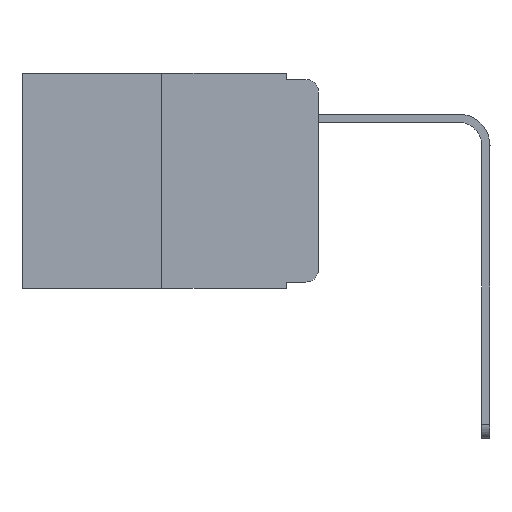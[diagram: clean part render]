
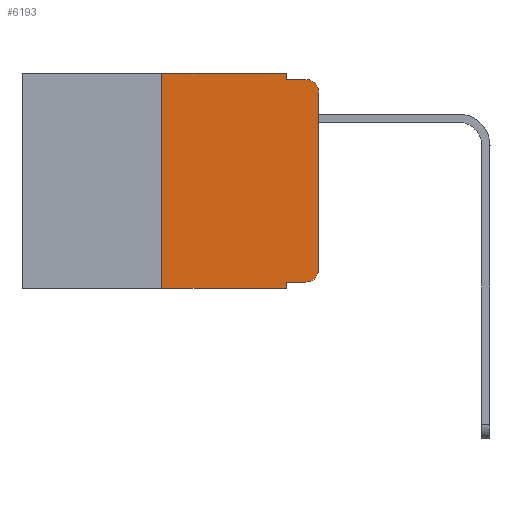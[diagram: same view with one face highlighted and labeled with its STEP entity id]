
A CAD part, left-side view. The second image highlights one B-rep face of the part: STEP entity #6193.
In plain terms, the highlighted planar face has unit normal (-1, 0, 0).
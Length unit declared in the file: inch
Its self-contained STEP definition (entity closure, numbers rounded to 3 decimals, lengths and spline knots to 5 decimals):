
#42 = LINE ( 'NONE', #4473, #7339 ) ;
#192 = CARTESIAN_POINT ( 'NONE',  ( 0., 0., -0.313 ) ) ;
#453 = DIRECTION ( 'NONE',  ( 0., -1., 0. ) ) ;
#806 = PLANE ( 'NONE',  #13889 ) ;
#850 = EDGE_CURVE ( 'NONE', #6566, #1438, #13291, .T. ) ;
#931 = DIRECTION ( 'NONE',  ( 0., 0., -1. ) ) ;
#1097 = ORIENTED_EDGE ( 'NONE', *, *, #3988, .F. ) ;
#1257 = ORIENTED_EDGE ( 'NONE', *, *, #9052, .F. ) ;
#1425 = ORIENTED_EDGE ( 'NONE', *, *, #13205, .F. ) ;
#1438 = VERTEX_POINT ( 'NONE', #192 ) ;
#2162 = CARTESIAN_POINT ( 'NONE',  ( 0., 0.051, -0.333 ) ) ;
#2212 = VERTEX_POINT ( 'NONE', #12755 ) ;
#2245 = CARTESIAN_POINT ( 'NONE',  ( 0., 0., -0.03 ) ) ;
#2748 = AXIS2_PLACEMENT_3D ( 'NONE', #15399, #9137, #2895 ) ;
#2895 = DIRECTION ( 'NONE',  ( 0., 0., -1. ) ) ;
#3057 = VERTEX_POINT ( 'NONE', #2162 ) ;
#3129 = EDGE_CURVE ( 'NONE', #2212, #14127, #7512, .T. ) ;
#3177 = CARTESIAN_POINT ( 'NONE',  ( 0., 0.25, 0. ) ) ;
#3271 = DIRECTION ( 'NONE',  ( 0., -1., 0. ) ) ;
#3306 = LINE ( 'NONE', #5406, #7993 ) ;
#3517 = EDGE_CURVE ( 'NONE', #1438, #9092, #13739, .T. ) ;
#3805 = CARTESIAN_POINT ( 'NONE',  ( 0., 0.051, 0. ) ) ;
#3937 = VECTOR ( 'NONE', #11449, 39.37008 ) ;
#3988 = EDGE_CURVE ( 'NONE', #9483, #11467, #14746, .T. ) ;
#4106 = VECTOR ( 'NONE', #14492, 39.37008 ) ;
#4350 = VECTOR ( 'NONE', #3271, 39.37008 ) ;
#4447 = EDGE_LOOP ( 'NONE', ( #4519, #15359, #1425, #10520, #1097, #1257, #13998, #5486, #8314, #6556 ) ) ;
#4473 = CARTESIAN_POINT ( 'NONE',  ( 0., 0.051, 0. ) ) ;
#4491 = CARTESIAN_POINT ( 'NONE',  ( 0., 0.25, 0. ) ) ;
#4519 = ORIENTED_EDGE ( 'NONE', *, *, #3517, .T. ) ;
#4652 = EDGE_CURVE ( 'NONE', #3057, #6566, #5117, .T. ) ;
#5107 = CARTESIAN_POINT ( 'NONE',  ( 0., 0.051, 0. ) ) ;
#5117 = LINE ( 'NONE', #9577, #4106 ) ;
#5406 = CARTESIAN_POINT ( 'NONE',  ( 0., 0.051, -0.01 ) ) ;
#5486 = ORIENTED_EDGE ( 'NONE', *, *, #9436, .F. ) ;
#5592 = VERTEX_POINT ( 'NONE', #7931 ) ;
#5641 = CARTESIAN_POINT ( 'NONE',  ( 0., 0.473, 0. ) ) ;
#5762 = VECTOR ( 'NONE', #6874, 39.37008 ) ;
#5897 = CARTESIAN_POINT ( 'NONE',  ( 0., 0.02, -0.01 ) ) ;
#6193 = ADVANCED_FACE ( 'NONE', ( #12521 ), #806, .F. ) ;
#6324 = VECTOR ( 'NONE', #10556, 39.37008 ) ;
#6556 = ORIENTED_EDGE ( 'NONE', *, *, #850, .T. ) ;
#6566 = VERTEX_POINT ( 'NONE', #15371 ) ;
#6835 = CIRCLE ( 'NONE', #2748, 0.02 ) ;
#6874 = DIRECTION ( 'NONE',  ( 0., 0., 1. ) ) ;
#6930 = AXIS2_PLACEMENT_3D ( 'NONE', #10296, #10201, #15244 ) ;
#7339 = VECTOR ( 'NONE', #10279, 39.37008 ) ;
#7512 = LINE ( 'NONE', #14493, #4350 ) ;
#7931 = CARTESIAN_POINT ( 'NONE',  ( 0., 0.051, -0.01 ) ) ;
#7993 = VECTOR ( 'NONE', #453, 39.37008 ) ;
#8124 = LINE ( 'NONE', #4491, #13773 ) ;
#8314 = ORIENTED_EDGE ( 'NONE', *, *, #4652, .T. ) ;
#8743 = VERTEX_POINT ( 'NONE', #5897 ) ;
#9052 = EDGE_CURVE ( 'NONE', #2212, #9483, #8124, .T. ) ;
#9092 = VERTEX_POINT ( 'NONE', #2245 ) ;
#9137 = DIRECTION ( 'NONE',  ( -1., 0., 0. ) ) ;
#9436 = EDGE_CURVE ( 'NONE', #3057, #14127, #42, .T. ) ;
#9483 = VERTEX_POINT ( 'NONE', #3177 ) ;
#9506 = CARTESIAN_POINT ( 'NONE',  ( 0., 0.473, 0. ) ) ;
#9561 = DIRECTION ( 'NONE',  ( 1., 0., 0. ) ) ;
#9577 = CARTESIAN_POINT ( 'NONE',  ( 0., 0.051, -0.333 ) ) ;
#10201 = DIRECTION ( 'NONE',  ( -1., 0., 0. ) ) ;
#10279 = DIRECTION ( 'NONE',  ( 0., 0., -1. ) ) ;
#10296 = CARTESIAN_POINT ( 'NONE',  ( 0., 0.02, -0.313 ) ) ;
#10520 = ORIENTED_EDGE ( 'NONE', *, *, #10917, .F. ) ;
#10556 = DIRECTION ( 'NONE',  ( 0., -1., 0. ) ) ;
#10917 = EDGE_CURVE ( 'NONE', #11467, #5592, #15736, .T. ) ;
#11449 = DIRECTION ( 'NONE',  ( 0., 0., -1. ) ) ;
#11467 = VERTEX_POINT ( 'NONE', #5107 ) ;
#12521 = FACE_OUTER_BOUND ( 'NONE', #4447, .T. ) ;
#12755 = CARTESIAN_POINT ( 'NONE',  ( 0., 0.25, -0.343 ) ) ;
#13205 = EDGE_CURVE ( 'NONE', #5592, #8743, #3306, .T. ) ;
#13231 = EDGE_CURVE ( 'NONE', #9092, #8743, #6835, .T. ) ;
#13291 = CIRCLE ( 'NONE', #6930, 0.02 ) ;
#13739 = LINE ( 'NONE', #15365, #5762 ) ;
#13773 = VECTOR ( 'NONE', #15972, 39.37008 ) ;
#13889 = AXIS2_PLACEMENT_3D ( 'NONE', #9506, #9561, #931 ) ;
#13998 = ORIENTED_EDGE ( 'NONE', *, *, #3129, .T. ) ;
#14127 = VERTEX_POINT ( 'NONE', #15985 ) ;
#14492 = DIRECTION ( 'NONE',  ( 0., -1., 0. ) ) ;
#14493 = CARTESIAN_POINT ( 'NONE',  ( 0., 0.473, -0.343 ) ) ;
#14746 = LINE ( 'NONE', #5641, #6324 ) ;
#15244 = DIRECTION ( 'NONE',  ( 0., 0., -1. ) ) ;
#15359 = ORIENTED_EDGE ( 'NONE', *, *, #13231, .T. ) ;
#15365 = CARTESIAN_POINT ( 'NONE',  ( 0., 0., 0. ) ) ;
#15371 = CARTESIAN_POINT ( 'NONE',  ( 0., 0.02, -0.333 ) ) ;
#15399 = CARTESIAN_POINT ( 'NONE',  ( 0., 0.02, -0.03 ) ) ;
#15736 = LINE ( 'NONE', #3805, #3937 ) ;
#15972 = DIRECTION ( 'NONE',  ( 0., 0., 1. ) ) ;
#15985 = CARTESIAN_POINT ( 'NONE',  ( 0., 0.051, -0.343 ) ) ;
